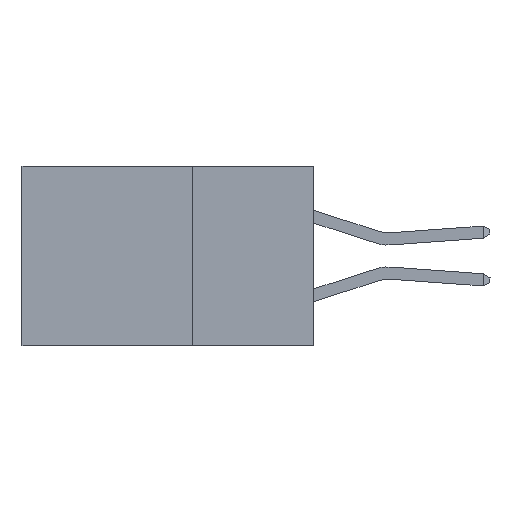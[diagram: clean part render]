
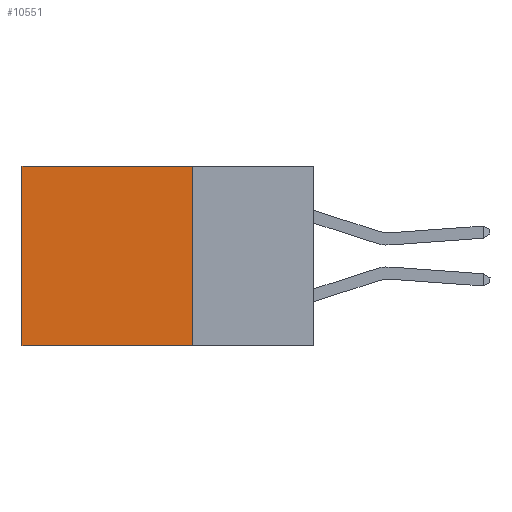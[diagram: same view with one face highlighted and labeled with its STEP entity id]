
A CAD part, left-side view. The second image highlights one B-rep face of the part: STEP entity #10551.
In plain terms, the highlighted planar face has unit normal (-1, 0, 0).
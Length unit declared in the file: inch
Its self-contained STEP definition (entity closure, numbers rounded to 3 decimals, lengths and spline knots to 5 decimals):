
#1110 = CARTESIAN_POINT ( 'NONE',  ( 0.2875, 0.6, 0. ) ) ;
#1146 = LINE ( 'NONE', #3122, #5851 ) ;
#2105 = CARTESIAN_POINT ( 'NONE',  ( 0.2875, 0.25, -0.37 ) ) ;
#2810 = EDGE_CURVE ( 'NONE', #10857, #11131, #1146, .T. ) ;
#3020 = DIRECTION ( 'NONE',  ( 0., 1., 0. ) ) ;
#3122 = CARTESIAN_POINT ( 'NONE',  ( 0.2875, 0.25, 0. ) ) ;
#3282 = AXIS2_PLACEMENT_3D ( 'NONE', #10527, #5227, #11389 ) ;
#3375 = VECTOR ( 'NONE', #7288, 39.37008 ) ;
#3379 = LINE ( 'NONE', #10140, #8040 ) ;
#3409 = EDGE_CURVE ( 'NONE', #10857, #4533, #3379, .T. ) ;
#3475 = PLANE ( 'NONE',  #3282 ) ;
#3929 = VECTOR ( 'NONE', #3020, 39.37008 ) ;
#4004 = EDGE_CURVE ( 'NONE', #4533, #8059, #6263, .T. ) ;
#4280 = ORIENTED_EDGE ( 'NONE', *, *, #4004, .F. ) ;
#4515 = EDGE_CURVE ( 'NONE', #11131, #8059, #5415, .T. ) ;
#4533 = VERTEX_POINT ( 'NONE', #10865 ) ;
#4553 = ORIENTED_EDGE ( 'NONE', *, *, #3409, .F. ) ;
#5227 = DIRECTION ( 'NONE',  ( 1., 0., 0. ) ) ;
#5236 = CARTESIAN_POINT ( 'NONE',  ( 0.2875, 0.6, -0.37 ) ) ;
#5415 = LINE ( 'NONE', #1110, #3375 ) ;
#5637 = EDGE_LOOP ( 'NONE', ( #8403, #4280, #4553, #6487 ) ) ;
#5851 = VECTOR ( 'NONE', #8378, 39.37008 ) ;
#6263 = LINE ( 'NONE', #2105, #3929 ) ;
#6487 = ORIENTED_EDGE ( 'NONE', *, *, #2810, .T. ) ;
#7006 = CARTESIAN_POINT ( 'NONE',  ( 0.2875, 0.25, 0. ) ) ;
#7288 = DIRECTION ( 'NONE',  ( 0., 0., -1. ) ) ;
#8040 = VECTOR ( 'NONE', #11029, 39.37008 ) ;
#8059 = VERTEX_POINT ( 'NONE', #5236 ) ;
#8378 = DIRECTION ( 'NONE',  ( 0., 1., 0. ) ) ;
#8403 = ORIENTED_EDGE ( 'NONE', *, *, #4515, .T. ) ;
#10085 = CARTESIAN_POINT ( 'NONE',  ( 0.2875, 0.6, 0. ) ) ;
#10140 = CARTESIAN_POINT ( 'NONE',  ( 0.2875, 0.25, 0. ) ) ;
#10527 = CARTESIAN_POINT ( 'NONE',  ( 0.2875, 0.25, 0. ) ) ;
#10551 = ADVANCED_FACE ( 'NONE', ( #10627 ), #3475, .F. ) ;
#10627 = FACE_OUTER_BOUND ( 'NONE', #5637, .T. ) ;
#10857 = VERTEX_POINT ( 'NONE', #7006 ) ;
#10865 = CARTESIAN_POINT ( 'NONE',  ( 0.2875, 0.25, -0.37 ) ) ;
#11029 = DIRECTION ( 'NONE',  ( 0., 0., -1. ) ) ;
#11131 = VERTEX_POINT ( 'NONE', #10085 ) ;
#11389 = DIRECTION ( 'NONE',  ( 0., 0., -1. ) ) ;
